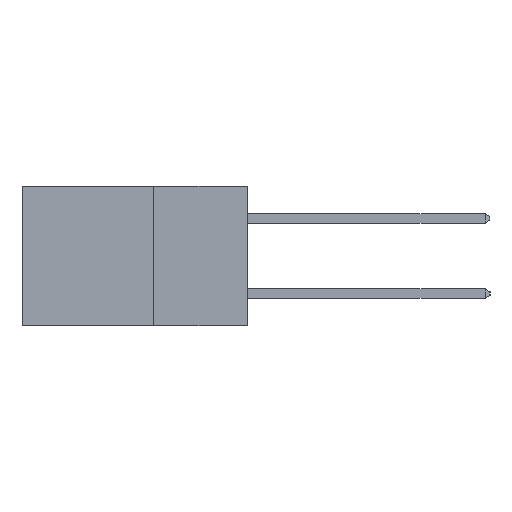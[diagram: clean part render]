
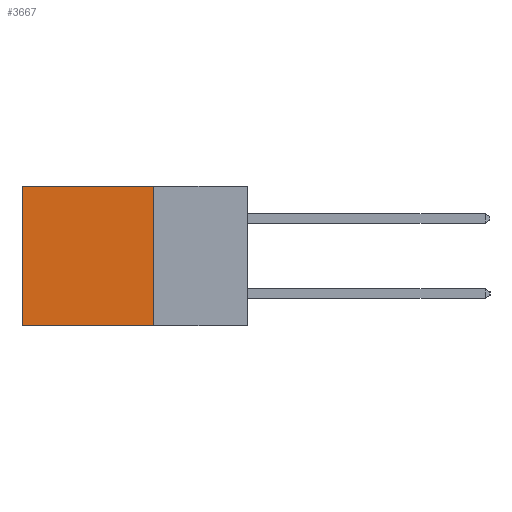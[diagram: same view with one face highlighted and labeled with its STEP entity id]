
A CAD part, left-side view. The second image highlights one B-rep face of the part: STEP entity #3667.
In plain terms, the highlighted planar face has unit normal (-1, 0, 0).
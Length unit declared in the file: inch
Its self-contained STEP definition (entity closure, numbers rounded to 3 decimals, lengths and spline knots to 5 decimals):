
#203 = VECTOR ( 'NONE', #4386, 39.37008 ) ;
#698 = VECTOR ( 'NONE', #8965, 39.37008 ) ;
#957 = EDGE_CURVE ( 'NONE', #4206, #5236, #1347, .T. ) ;
#1347 = LINE ( 'NONE', #8869, #8558 ) ;
#1426 = FACE_OUTER_BOUND ( 'NONE', #8308, .T. ) ;
#1762 = CARTESIAN_POINT ( 'NONE',  ( 0.2615, 0.25, -0.37 ) ) ;
#1864 = DIRECTION ( 'NONE',  ( 1., 0., 0. ) ) ;
#1879 = DIRECTION ( 'NONE',  ( 0., 0., -1. ) ) ;
#2230 = PLANE ( 'NONE',  #4737 ) ;
#2396 = DIRECTION ( 'NONE',  ( 0., 0., -1. ) ) ;
#2474 = CARTESIAN_POINT ( 'NONE',  ( 0.2615, 0.6, -0.37 ) ) ;
#2751 = VERTEX_POINT ( 'NONE', #2474 ) ;
#2995 = CARTESIAN_POINT ( 'NONE',  ( 0.2615, 0.25, 0. ) ) ;
#3150 = ORIENTED_EDGE ( 'NONE', *, *, #3197, .F. ) ;
#3197 = EDGE_CURVE ( 'NONE', #3372, #2751, #8626, .T. ) ;
#3372 = VERTEX_POINT ( 'NONE', #4680 ) ;
#3667 = ADVANCED_FACE ( 'NONE', ( #1426 ), #2230, .F. ) ;
#3844 = ORIENTED_EDGE ( 'NONE', *, *, #6146, .F. ) ;
#4206 = VERTEX_POINT ( 'NONE', #2995 ) ;
#4386 = DIRECTION ( 'NONE',  ( 0., 0., -1. ) ) ;
#4401 = CARTESIAN_POINT ( 'NONE',  ( 0.2615, 0.6, -0.37 ) ) ;
#4680 = CARTESIAN_POINT ( 'NONE',  ( 0.2615, 0.25, -0.37 ) ) ;
#4737 = AXIS2_PLACEMENT_3D ( 'NONE', #7469, #1864, #2396 ) ;
#5236 = VERTEX_POINT ( 'NONE', #7242 ) ;
#5476 = EDGE_CURVE ( 'NONE', #5236, #2751, #5913, .T. ) ;
#5831 = CARTESIAN_POINT ( 'NONE',  ( 0.2615, 0.25, -0.37 ) ) ;
#5913 = LINE ( 'NONE', #4401, #203 ) ;
#6146 = EDGE_CURVE ( 'NONE', #4206, #3372, #7809, .T. ) ;
#6269 = ORIENTED_EDGE ( 'NONE', *, *, #957, .T. ) ;
#6272 = ORIENTED_EDGE ( 'NONE', *, *, #5476, .T. ) ;
#7242 = CARTESIAN_POINT ( 'NONE',  ( 0.2615, 0.6, 0. ) ) ;
#7469 = CARTESIAN_POINT ( 'NONE',  ( 0.2615, 0.25, -0.37 ) ) ;
#7809 = LINE ( 'NONE', #1762, #9447 ) ;
#8176 = DIRECTION ( 'NONE',  ( 0., 1., 0. ) ) ;
#8308 = EDGE_LOOP ( 'NONE', ( #6272, #3150, #3844, #6269 ) ) ;
#8558 = VECTOR ( 'NONE', #8176, 39.37008 ) ;
#8626 = LINE ( 'NONE', #5831, #698 ) ;
#8869 = CARTESIAN_POINT ( 'NONE',  ( 0.2615, 0.25, 0. ) ) ;
#8965 = DIRECTION ( 'NONE',  ( 0., 1., 0. ) ) ;
#9447 = VECTOR ( 'NONE', #1879, 39.37008 ) ;
